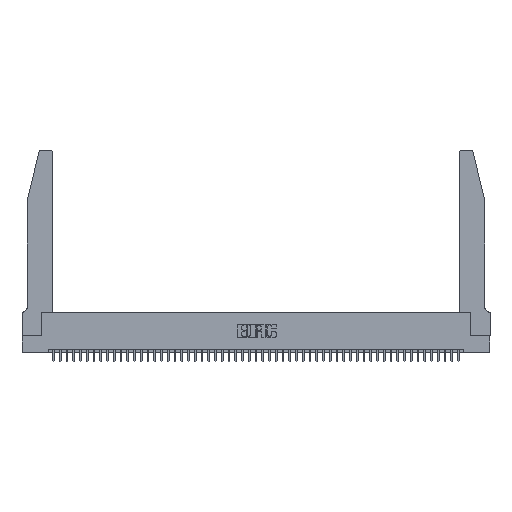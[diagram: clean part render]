
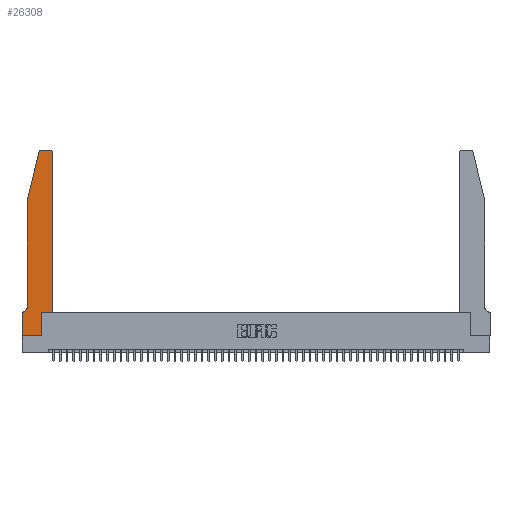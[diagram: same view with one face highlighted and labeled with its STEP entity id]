
A CAD part, top view. The second image highlights one B-rep face of the part: STEP entity #26308.
In plain terms, the highlighted planar face has unit normal (0, 0, 1).
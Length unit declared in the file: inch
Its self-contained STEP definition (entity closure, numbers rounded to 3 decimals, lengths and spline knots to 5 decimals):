
#1404 = LINE ( 'NONE', #22772, #21937 ) ;
#1672 = VERTEX_POINT ( 'NONE', #2188 ) ;
#1849 = LINE ( 'NONE', #35141, #8493 ) ;
#2053 = CARTESIAN_POINT ( 'NONE',  ( 0.4505, 0.35, 0.37 ) ) ;
#2188 = CARTESIAN_POINT ( 'NONE',  ( 0.284, 2.75, 0.37 ) ) ;
#2593 = VERTEX_POINT ( 'NONE', #36803 ) ;
#2940 = DIRECTION ( 'NONE',  ( 0., 0., 1. ) ) ;
#3085 = ORIENTED_EDGE ( 'NONE', *, *, #44058, .T. ) ;
#3371 = ORIENTED_EDGE ( 'NONE', *, *, #4800, .T. ) ;
#3726 = DIRECTION ( 'NONE',  ( 1., 0., 0. ) ) ;
#4800 = EDGE_CURVE ( 'NONE', #25558, #40273, #50009, .T. ) ;
#5428 = EDGE_CURVE ( 'NONE', #47422, #28766, #19103, .T. ) ;
#5619 = DIRECTION ( 'NONE',  ( 1., 0., 0. ) ) ;
#7263 = CARTESIAN_POINT ( 'NONE',  ( 0.4505, 2.72, 0.37 ) ) ;
#7885 = VERTEX_POINT ( 'NONE', #39972 ) ;
#8004 = CARTESIAN_POINT ( 'NONE',  ( 0.0755, 2., 0.37 ) ) ;
#8493 = VECTOR ( 'NONE', #23490, 39.37008 ) ;
#8877 = ORIENTED_EDGE ( 'NONE', *, *, #5428, .T. ) ;
#9142 = DIRECTION ( 'NONE',  ( 1., 0., 0. ) ) ;
#9786 = CARTESIAN_POINT ( 'NONE',  ( 0.2865, 0., 0.37 ) ) ;
#10019 = ORIENTED_EDGE ( 'NONE', *, *, #38172, .T. ) ;
#10234 = DIRECTION ( 'NONE',  ( -1., 0., 0. ) ) ;
#10704 = VECTOR ( 'NONE', #16383, 39.37008 ) ;
#10885 = CARTESIAN_POINT ( 'NONE',  ( 0.4505, 0.35, 0.37 ) ) ;
#11172 = AXIS2_PLACEMENT_3D ( 'NONE', #17414, #47851, #25113 ) ;
#11335 = DIRECTION ( 'NONE',  ( 0., 0., 1. ) ) ;
#11461 = VERTEX_POINT ( 'NONE', #30008 ) ;
#12681 = ORIENTED_EDGE ( 'NONE', *, *, #38236, .T. ) ;
#13725 = ORIENTED_EDGE ( 'NONE', *, *, #44886, .T. ) ;
#13778 = LINE ( 'NONE', #14800, #35480 ) ;
#14210 = VECTOR ( 'NONE', #10234, 39.37008 ) ;
#14549 = ORIENTED_EDGE ( 'NONE', *, *, #37082, .T. ) ;
#14800 = CARTESIAN_POINT ( 'NONE',  ( 0., 0., 0.37 ) ) ;
#15242 = DIRECTION ( 'NONE',  ( 1., 0., 0. ) ) ;
#15721 = DIRECTION ( 'NONE',  ( 0., 1., 0. ) ) ;
#16141 = VECTOR ( 'NONE', #27700, 39.37008 ) ;
#16383 = DIRECTION ( 'NONE',  ( 0., 1., 0. ) ) ;
#16750 = CARTESIAN_POINT ( 'NONE',  ( 0., 0., 0.37 ) ) ;
#17180 = ORIENTED_EDGE ( 'NONE', *, *, #46981, .T. ) ;
#17414 = CARTESIAN_POINT ( 'NONE',  ( 0.0055, 0.42, 0.37 ) ) ;
#17575 = AXIS2_PLACEMENT_3D ( 'NONE', #38479, #11335, #15242 ) ;
#17903 = CIRCLE ( 'NONE', #11172, 0.07 ) ;
#18423 = LINE ( 'NONE', #33317, #14210 ) ;
#18495 = PLANE ( 'NONE',  #18763 ) ;
#18658 = CARTESIAN_POINT ( 'NONE',  ( 0., 0.35, 0.37 ) ) ;
#18763 = AXIS2_PLACEMENT_3D ( 'NONE', #18658, #2940, #49438 ) ;
#19012 = CARTESIAN_POINT ( 'NONE',  ( 0., 0., 0.37 ) ) ;
#19103 = CIRCLE ( 'NONE', #17575, 0.03 ) ;
#19273 = CARTESIAN_POINT ( 'NONE',  ( 0.284, 2.72, 0.37 ) ) ;
#19505 = VERTEX_POINT ( 'NONE', #24183 ) ;
#21937 = VECTOR ( 'NONE', #15721, 39.37008 ) ;
#22011 = CARTESIAN_POINT ( 'NONE',  ( 0.2605, 2.75, 0.37 ) ) ;
#22036 = VERTEX_POINT ( 'NONE', #10885 ) ;
#22147 = LINE ( 'NONE', #8004, #16141 ) ;
#22336 = DIRECTION ( 'NONE',  ( -1., 0., 0. ) ) ;
#22772 = CARTESIAN_POINT ( 'NONE',  ( 0.4505, 0.35, 0.37 ) ) ;
#23490 = DIRECTION ( 'NONE',  ( 0., -1., 0. ) ) ;
#24183 = CARTESIAN_POINT ( 'NONE',  ( 0.0755, 0.42, 0.37 ) ) ;
#25113 = DIRECTION ( 'NONE',  ( -1., 0., 0. ) ) ;
#25321 = VECTOR ( 'NONE', #5619, 39.37008 ) ;
#25558 = VERTEX_POINT ( 'NONE', #9786 ) ;
#26308 = ADVANCED_FACE ( 'NONE', ( #43579 ), #18495, .T. ) ;
#26473 = CARTESIAN_POINT ( 'NONE',  ( 0., 0.35, 0.37 ) ) ;
#26790 = EDGE_CURVE ( 'NONE', #40273, #22036, #36248, .T. ) ;
#27028 = EDGE_CURVE ( 'NONE', #1672, #11461, #39828, .T. ) ;
#27700 = DIRECTION ( 'NONE',  ( -0.239, -0.971, 0. ) ) ;
#28766 = VERTEX_POINT ( 'NONE', #44531 ) ;
#29031 = VERTEX_POINT ( 'NONE', #26473 ) ;
#30008 = CARTESIAN_POINT ( 'NONE',  ( 0.25487, 2.72718, 0.37 ) ) ;
#30303 = VERTEX_POINT ( 'NONE', #19012 ) ;
#30439 = EDGE_LOOP ( 'NONE', ( #3085, #32856, #12681, #17180, #14549, #41888, #10019, #46613, #3371, #34178, #13725, #8877 ) ) ;
#31474 = EDGE_CURVE ( 'NONE', #2593, #29031, #18423, .T. ) ;
#32856 = ORIENTED_EDGE ( 'NONE', *, *, #27028, .T. ) ;
#33317 = CARTESIAN_POINT ( 'NONE',  ( 0.0755, 0.35, 0.37 ) ) ;
#33485 = VECTOR ( 'NONE', #22336, 39.37008 ) ;
#34178 = ORIENTED_EDGE ( 'NONE', *, *, #26790, .T. ) ;
#34645 = VECTOR ( 'NONE', #9142, 39.37008 ) ;
#34747 = CARTESIAN_POINT ( 'NONE',  ( 0.2865, 0.35, 0.37 ) ) ;
#35141 = CARTESIAN_POINT ( 'NONE',  ( 0.0755, 2., 0.37 ) ) ;
#35480 = VECTOR ( 'NONE', #46554, 39.37008 ) ;
#36248 = LINE ( 'NONE', #2053, #25321 ) ;
#36803 = CARTESIAN_POINT ( 'NONE',  ( 0.0055, 0.35, 0.37 ) ) ;
#37082 = EDGE_CURVE ( 'NONE', #19505, #2593, #17903, .T. ) ;
#38172 = EDGE_CURVE ( 'NONE', #29031, #30303, #13778, .T. ) ;
#38236 = EDGE_CURVE ( 'NONE', #11461, #7885, #22147, .T. ) ;
#38479 = CARTESIAN_POINT ( 'NONE',  ( 0.4205, 2.72, 0.37 ) ) ;
#39551 = LINE ( 'NONE', #22011, #33485 ) ;
#39828 = CIRCLE ( 'NONE', #46001, 0.03 ) ;
#39960 = EDGE_CURVE ( 'NONE', #30303, #25558, #48019, .T. ) ;
#39972 = CARTESIAN_POINT ( 'NONE',  ( 0.0755, 2., 0.37 ) ) ;
#40273 = VERTEX_POINT ( 'NONE', #34747 ) ;
#41888 = ORIENTED_EDGE ( 'NONE', *, *, #31474, .T. ) ;
#42928 = DIRECTION ( 'NONE',  ( 0., 0., 1. ) ) ;
#43078 = CARTESIAN_POINT ( 'NONE',  ( 0.2865, 0.35, 0.37 ) ) ;
#43579 = FACE_OUTER_BOUND ( 'NONE', #30439, .T. ) ;
#44058 = EDGE_CURVE ( 'NONE', #28766, #1672, #39551, .T. ) ;
#44531 = CARTESIAN_POINT ( 'NONE',  ( 0.4205, 2.75, 0.37 ) ) ;
#44886 = EDGE_CURVE ( 'NONE', #22036, #47422, #1404, .T. ) ;
#46001 = AXIS2_PLACEMENT_3D ( 'NONE', #19273, #42928, #3726 ) ;
#46554 = DIRECTION ( 'NONE',  ( 0., -1., 0. ) ) ;
#46613 = ORIENTED_EDGE ( 'NONE', *, *, #39960, .T. ) ;
#46981 = EDGE_CURVE ( 'NONE', #7885, #19505, #1849, .T. ) ;
#47422 = VERTEX_POINT ( 'NONE', #7263 ) ;
#47851 = DIRECTION ( 'NONE',  ( 0., 0., -1. ) ) ;
#48019 = LINE ( 'NONE', #16750, #34645 ) ;
#49438 = DIRECTION ( 'NONE',  ( 1., 0., 0. ) ) ;
#50009 = LINE ( 'NONE', #43078, #10704 ) ;
